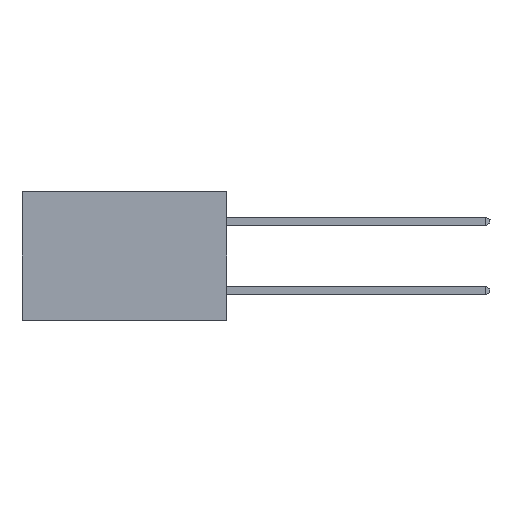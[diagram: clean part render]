
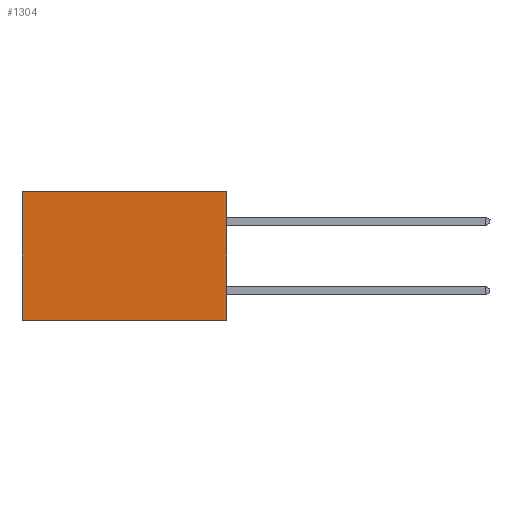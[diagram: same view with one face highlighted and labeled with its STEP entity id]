
A CAD part, left-side view. The second image highlights one B-rep face of the part: STEP entity #1304.
In plain terms, the highlighted planar face has unit normal (-1, 0, 0).
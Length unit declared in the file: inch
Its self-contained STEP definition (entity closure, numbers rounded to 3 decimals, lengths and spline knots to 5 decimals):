
#220 = LINE ( 'NONE', #6453, #4634 ) ;
#1304 = ADVANCED_FACE ( 'NONE', ( #17963 ), #7174, .F. ) ;
#1650 = ORIENTED_EDGE ( 'NONE', *, *, #12835, .T. ) ;
#2146 = ORIENTED_EDGE ( 'NONE', *, *, #4425, .F. ) ;
#2581 = ORIENTED_EDGE ( 'NONE', *, *, #10337, .F. ) ;
#3468 = ORIENTED_EDGE ( 'NONE', *, *, #17218, .T. ) ;
#3655 = CARTESIAN_POINT ( 'NONE',  ( 0.277, 0.59, 0. ) ) ;
#3958 = DIRECTION ( 'NONE',  ( 0., 0., -1. ) ) ;
#4425 = EDGE_CURVE ( 'NONE', #8364, #8179, #6511, .T. ) ;
#4634 = VECTOR ( 'NONE', #6488, 39.37008 ) ;
#4915 = AXIS2_PLACEMENT_3D ( 'NONE', #9189, #7195, #3958 ) ;
#5403 = CARTESIAN_POINT ( 'NONE',  ( 0.277, 0., 0. ) ) ;
#6056 = VECTOR ( 'NONE', #15593, 39.37008 ) ;
#6453 = CARTESIAN_POINT ( 'NONE',  ( 0.277, 0., -0.37 ) ) ;
#6488 = DIRECTION ( 'NONE',  ( 0., 0., -1. ) ) ;
#6511 = LINE ( 'NONE', #15082, #6056 ) ;
#7174 = PLANE ( 'NONE',  #4915 ) ;
#7195 = DIRECTION ( 'NONE',  ( 1., 0., 0. ) ) ;
#8112 = EDGE_LOOP ( 'NONE', ( #1650, #2146, #2581, #3468 ) ) ;
#8179 = VERTEX_POINT ( 'NONE', #15999 ) ;
#8364 = VERTEX_POINT ( 'NONE', #14934 ) ;
#8813 = LINE ( 'NONE', #10388, #12620 ) ;
#9120 = LINE ( 'NONE', #16562, #12464 ) ;
#9189 = CARTESIAN_POINT ( 'NONE',  ( 0.277, 0., -0.37 ) ) ;
#10337 = EDGE_CURVE ( 'NONE', #15747, #8364, #220, .T. ) ;
#10352 = DIRECTION ( 'NONE',  ( 0., 0., -1. ) ) ;
#10388 = CARTESIAN_POINT ( 'NONE',  ( 0.277, 0.59, -0.37 ) ) ;
#10572 = VERTEX_POINT ( 'NONE', #3655 ) ;
#12464 = VECTOR ( 'NONE', #15439, 39.37008 ) ;
#12620 = VECTOR ( 'NONE', #10352, 39.37008 ) ;
#12835 = EDGE_CURVE ( 'NONE', #10572, #8179, #8813, .T. ) ;
#14934 = CARTESIAN_POINT ( 'NONE',  ( 0.277, 0., -0.37 ) ) ;
#15082 = CARTESIAN_POINT ( 'NONE',  ( 0.277, 0., -0.37 ) ) ;
#15439 = DIRECTION ( 'NONE',  ( 0., 1., 0. ) ) ;
#15593 = DIRECTION ( 'NONE',  ( 0., 1., 0. ) ) ;
#15747 = VERTEX_POINT ( 'NONE', #5403 ) ;
#15999 = CARTESIAN_POINT ( 'NONE',  ( 0.277, 0.59, -0.37 ) ) ;
#16562 = CARTESIAN_POINT ( 'NONE',  ( 0.277, 0., 0. ) ) ;
#17218 = EDGE_CURVE ( 'NONE', #15747, #10572, #9120, .T. ) ;
#17963 = FACE_OUTER_BOUND ( 'NONE', #8112, .T. ) ;
